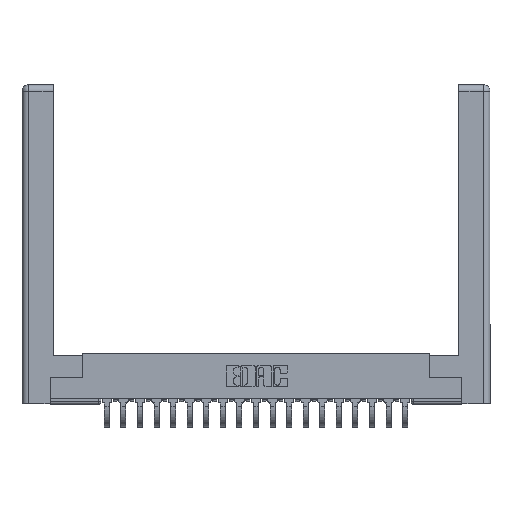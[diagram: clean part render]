
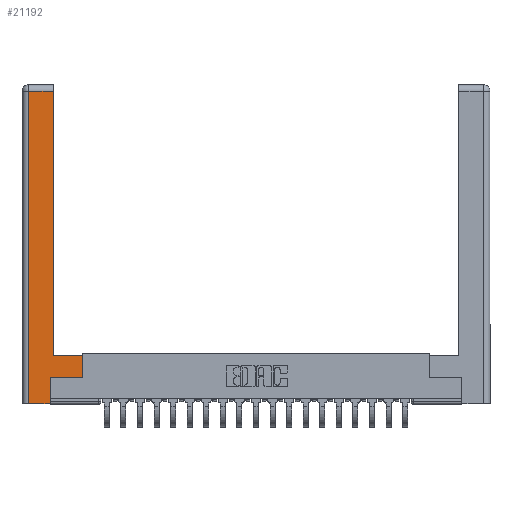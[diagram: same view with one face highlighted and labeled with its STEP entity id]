
A CAD part, top view. The second image highlights one B-rep face of the part: STEP entity #21192.
In plain terms, the highlighted planar face has unit normal (0, 0, 1).
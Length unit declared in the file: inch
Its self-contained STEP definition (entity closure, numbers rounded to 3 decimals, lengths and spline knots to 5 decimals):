
#263 = LINE ( 'NONE', #13287, #16219 ) ;
#589 = LINE ( 'NONE', #2742, #824 ) ;
#683 = EDGE_CURVE ( 'NONE', #23577, #16873, #7827, .T. ) ;
#824 = VECTOR ( 'NONE', #2634, 39.37008 ) ;
#1035 = EDGE_LOOP ( 'NONE', ( #2466, #14104, #14552, #7715, #19754, #19944, #19061, #3618 ) ) ;
#1242 = CARTESIAN_POINT ( 'NONE',  ( 0.265, 0.245, 0. ) ) ;
#1632 = VERTEX_POINT ( 'NONE', #10502 ) ;
#1715 = VECTOR ( 'NONE', #5892, 39.37008 ) ;
#2128 = FACE_OUTER_BOUND ( 'NONE', #1035, .T. ) ;
#2466 = ORIENTED_EDGE ( 'NONE', *, *, #19269, .T. ) ;
#2634 = DIRECTION ( 'NONE',  ( 0., -1., 0. ) ) ;
#2742 = CARTESIAN_POINT ( 'NONE',  ( 0.0615, 0., 0. ) ) ;
#2984 = CARTESIAN_POINT ( 'NONE',  ( 0.565, 0.45, 0. ) ) ;
#3033 = CARTESIAN_POINT ( 'NONE',  ( 0.295, 0.45, 0. ) ) ;
#3618 = ORIENTED_EDGE ( 'NONE', *, *, #683, .T. ) ;
#3771 = VERTEX_POINT ( 'NONE', #6810 ) ;
#4052 = DIRECTION ( 'NONE',  ( 0., 1., 0. ) ) ;
#4529 = EDGE_CURVE ( 'NONE', #7998, #9206, #263, .T. ) ;
#4747 = CARTESIAN_POINT ( 'NONE',  ( 0.0615, 0., 0. ) ) ;
#4825 = EDGE_CURVE ( 'NONE', #9206, #23577, #15953, .T. ) ;
#5162 = LINE ( 'NONE', #7577, #10477 ) ;
#5304 = VECTOR ( 'NONE', #21438, 39.37008 ) ;
#5892 = DIRECTION ( 'NONE',  ( -1., 0., 0. ) ) ;
#6239 = VERTEX_POINT ( 'NONE', #19843 ) ;
#6335 = VECTOR ( 'NONE', #10298, 39.37008 ) ;
#6571 = LINE ( 'NONE', #12129, #5304 ) ;
#6810 = CARTESIAN_POINT ( 'NONE',  ( 0.0615, 2.94, 0. ) ) ;
#7556 = LINE ( 'NONE', #16189, #10302 ) ;
#7577 = CARTESIAN_POINT ( 'NONE',  ( 0.265, 0., 0. ) ) ;
#7715 = ORIENTED_EDGE ( 'NONE', *, *, #23305, .T. ) ;
#7827 = LINE ( 'NONE', #15083, #1715 ) ;
#7998 = VERTEX_POINT ( 'NONE', #17666 ) ;
#8619 = EDGE_CURVE ( 'NONE', #3771, #11405, #589, .T. ) ;
#9016 = DIRECTION ( 'NONE',  ( 1., 0., 0. ) ) ;
#9206 = VERTEX_POINT ( 'NONE', #12699 ) ;
#9483 = PLANE ( 'NONE',  #15349 ) ;
#10298 = DIRECTION ( 'NONE',  ( 0., 1., 0. ) ) ;
#10302 = VECTOR ( 'NONE', #4052, 39.37008 ) ;
#10477 = VECTOR ( 'NONE', #9016, 39.37008 ) ;
#10502 = CARTESIAN_POINT ( 'NONE',  ( 0.295, 2.94, 0. ) ) ;
#11405 = VERTEX_POINT ( 'NONE', #4747 ) ;
#12129 = CARTESIAN_POINT ( 'NONE',  ( 0.0615, 2.94, 0. ) ) ;
#12699 = CARTESIAN_POINT ( 'NONE',  ( 0.565, 0.245, 0. ) ) ;
#12934 = DIRECTION ( 'NONE',  ( 1., 0., 0. ) ) ;
#13287 = CARTESIAN_POINT ( 'NONE',  ( 0.565, 0.245, 0. ) ) ;
#14104 = ORIENTED_EDGE ( 'NONE', *, *, #19694, .T. ) ;
#14552 = ORIENTED_EDGE ( 'NONE', *, *, #8619, .T. ) ;
#15083 = CARTESIAN_POINT ( 'NONE',  ( 0.295, 0.45, 0. ) ) ;
#15169 = DIRECTION ( 'NONE',  ( 0., 0., -1. ) ) ;
#15177 = EDGE_CURVE ( 'NONE', #6239, #7998, #19832, .T. ) ;
#15349 = AXIS2_PLACEMENT_3D ( 'NONE', #20832, #15169, #22408 ) ;
#15953 = LINE ( 'NONE', #17999, #22714 ) ;
#16189 = CARTESIAN_POINT ( 'NONE',  ( 0.295, 3., 0. ) ) ;
#16219 = VECTOR ( 'NONE', #12934, 39.37008 ) ;
#16873 = VERTEX_POINT ( 'NONE', #3033 ) ;
#17666 = CARTESIAN_POINT ( 'NONE',  ( 0.265, 0.245, 0. ) ) ;
#17999 = CARTESIAN_POINT ( 'NONE',  ( 0.565, 0.45, 0. ) ) ;
#19061 = ORIENTED_EDGE ( 'NONE', *, *, #4825, .T. ) ;
#19269 = EDGE_CURVE ( 'NONE', #16873, #1632, #7556, .T. ) ;
#19694 = EDGE_CURVE ( 'NONE', #1632, #3771, #6571, .T. ) ;
#19754 = ORIENTED_EDGE ( 'NONE', *, *, #15177, .T. ) ;
#19832 = LINE ( 'NONE', #1242, #6335 ) ;
#19843 = CARTESIAN_POINT ( 'NONE',  ( 0.265, 0., 0. ) ) ;
#19944 = ORIENTED_EDGE ( 'NONE', *, *, #4529, .T. ) ;
#20832 = CARTESIAN_POINT ( 'NONE',  ( 0., 0., 0. ) ) ;
#21192 = ADVANCED_FACE ( 'NONE', ( #2128 ), #9483, .F. ) ;
#21438 = DIRECTION ( 'NONE',  ( -1., 0., 0. ) ) ;
#21500 = DIRECTION ( 'NONE',  ( 0., 1., 0. ) ) ;
#22408 = DIRECTION ( 'NONE',  ( -1., 0., 0. ) ) ;
#22714 = VECTOR ( 'NONE', #21500, 39.37008 ) ;
#23305 = EDGE_CURVE ( 'NONE', #11405, #6239, #5162, .T. ) ;
#23577 = VERTEX_POINT ( 'NONE', #2984 ) ;
